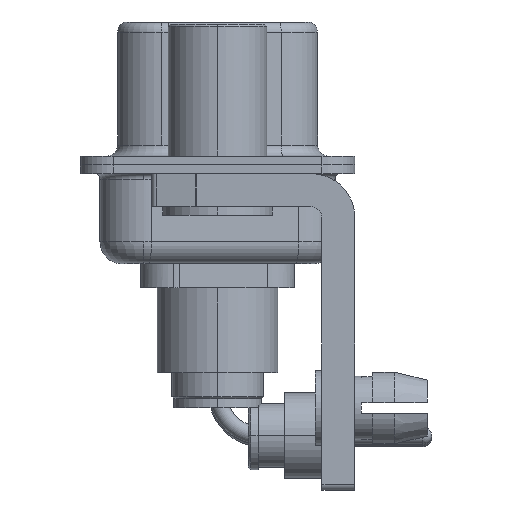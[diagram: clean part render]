
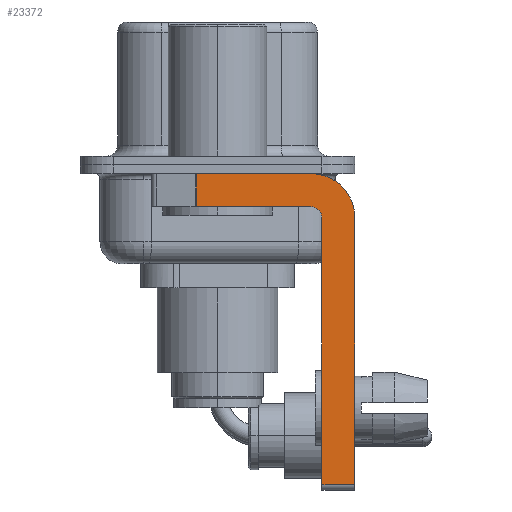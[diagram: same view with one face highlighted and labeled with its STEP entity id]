
A CAD part, left-side view. The second image highlights one B-rep face of the part: STEP entity #23372.
In plain terms, the highlighted planar face has unit normal (-1, 0, 0).
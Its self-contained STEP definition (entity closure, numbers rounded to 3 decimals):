
#220 = CARTESIAN_POINT ( 'NONE',  ( -2.9, -4.25, -1.9 ) ) ;
#683 = CARTESIAN_POINT ( 'NONE',  ( -2.9, -4.25, -2.4 ) ) ;
#1037 = CARTESIAN_POINT ( 'NONE',  ( -2.9, -4.75, -14.8 ) ) ;
#1614 = VERTEX_POINT ( 'NONE', #18601 ) ;
#1697 = DIRECTION ( 'NONE',  ( 0., 0., -1. ) ) ;
#1940 = ORIENTED_EDGE ( 'NONE', *, *, #13351, .T. ) ;
#2258 = DIRECTION ( 'NONE',  ( 0., -1., 0. ) ) ;
#2366 = VECTOR ( 'NONE', #3899, 1000. ) ;
#2411 = ORIENTED_EDGE ( 'NONE', *, *, #8951, .T. ) ;
#2453 = DIRECTION ( 'NONE',  ( 0., 0., -1. ) ) ;
#2888 = VECTOR ( 'NONE', #1697, 1000. ) ;
#3038 = CARTESIAN_POINT ( 'NONE',  ( -2.9, -4.75, -14.55 ) ) ;
#3170 = CARTESIAN_POINT ( 'NONE',  ( -2.9, -4.75, -2.4 ) ) ;
#3884 = CARTESIAN_POINT ( 'NONE',  ( -2.9, -4.25, -2.4 ) ) ;
#3899 = DIRECTION ( 'NONE',  ( 0., 1., 0. ) ) ;
#4109 = EDGE_LOOP ( 'NONE', ( #14324, #1940, #21962, #21634, #16506, #2411, #12765, #16739 ) ) ;
#4476 = LINE ( 'NONE', #1037, #23178 ) ;
#4547 = VERTEX_POINT ( 'NONE', #5367 ) ;
#4583 = CARTESIAN_POINT ( 'NONE',  ( -2.9, -6.25, -2.4 ) ) ;
#4943 = CARTESIAN_POINT ( 'NONE',  ( -2.9, -6.25, -2.4 ) ) ;
#5138 = CARTESIAN_POINT ( 'NONE',  ( -2.9, 0.978, -1.9 ) ) ;
#5247 = CARTESIAN_POINT ( 'NONE',  ( -2.9, -4.25, -2.4 ) ) ;
#5367 = CARTESIAN_POINT ( 'NONE',  ( -2.9, 0.978, -1.9 ) ) ;
#5424 = VERTEX_POINT ( 'NONE', #9056 ) ;
#6057 = VERTEX_POINT ( 'NONE', #7486 ) ;
#6517 = VECTOR ( 'NONE', #21369, 1000. ) ;
#7483 = AXIS2_PLACEMENT_3D ( 'NONE', #3884, #16546, #2453 ) ;
#7486 = CARTESIAN_POINT ( 'NONE',  ( -2.9, -4.25, -1.9 ) ) ;
#7916 = DIRECTION ( 'NONE',  ( -1., 0., 0. ) ) ;
#8078 = EDGE_CURVE ( 'NONE', #6057, #4547, #18110, .T. ) ;
#8243 = EDGE_CURVE ( 'NONE', #18488, #8383, #4476, .T. ) ;
#8383 = VERTEX_POINT ( 'NONE', #3170 ) ;
#8951 = EDGE_CURVE ( 'NONE', #18488, #5424, #23147, .T. ) ;
#9040 = DIRECTION ( 'NONE',  ( 0., 0., -1. ) ) ;
#9056 = CARTESIAN_POINT ( 'NONE',  ( -2.9, -6.25, -14.55 ) ) ;
#9406 = VERTEX_POINT ( 'NONE', #12655 ) ;
#9468 = DIRECTION ( 'NONE',  ( 0., 0., 1. ) ) ;
#10179 = AXIS2_PLACEMENT_3D ( 'NONE', #5247, #23237, #9040 ) ;
#10698 = PLANE ( 'NONE',  #10179 ) ;
#11589 = EDGE_CURVE ( 'NONE', #16038, #5424, #12169, .T. ) ;
#12169 = LINE ( 'NONE', #4943, #21726 ) ;
#12655 = CARTESIAN_POINT ( 'NONE',  ( -2.9, -4.25, -0.4 ) ) ;
#12765 = ORIENTED_EDGE ( 'NONE', *, *, #11589, .F. ) ;
#13351 = EDGE_CURVE ( 'NONE', #1614, #4547, #21689, .T. ) ;
#13500 = VECTOR ( 'NONE', #2258, 1000. ) ;
#14148 = CARTESIAN_POINT ( 'NONE',  ( -2.9, -4.25, -14.55 ) ) ;
#14324 = ORIENTED_EDGE ( 'NONE', *, *, #21709, .F. ) ;
#15143 = LINE ( 'NONE', #16702, #13500 ) ;
#15465 = DIRECTION ( 'NONE',  ( 0., 0., -1. ) ) ;
#15849 = EDGE_CURVE ( 'NONE', #9406, #16038, #17685, .T. ) ;
#16038 = VERTEX_POINT ( 'NONE', #4583 ) ;
#16506 = ORIENTED_EDGE ( 'NONE', *, *, #8243, .F. ) ;
#16546 = DIRECTION ( 'NONE',  ( 1., 0., 0. ) ) ;
#16702 = CARTESIAN_POINT ( 'NONE',  ( -2.9, 3., -0.4 ) ) ;
#16739 = ORIENTED_EDGE ( 'NONE', *, *, #15849, .F. ) ;
#17302 = CIRCLE ( 'NONE', #20344, 0.5 ) ;
#17685 = CIRCLE ( 'NONE', #7483, 2. ) ;
#18110 = LINE ( 'NONE', #220, #2366 ) ;
#18488 = VERTEX_POINT ( 'NONE', #3038 ) ;
#18601 = CARTESIAN_POINT ( 'NONE',  ( -2.9, 0.978, -0.4 ) ) ;
#19917 = FACE_OUTER_BOUND ( 'NONE', #4109, .T. ) ;
#20344 = AXIS2_PLACEMENT_3D ( 'NONE', #683, #7916, #9468 ) ;
#21369 = DIRECTION ( 'NONE',  ( 0., -1., 0. ) ) ;
#21634 = ORIENTED_EDGE ( 'NONE', *, *, #22163, .F. ) ;
#21689 = LINE ( 'NONE', #5138, #2888 ) ;
#21709 = EDGE_CURVE ( 'NONE', #1614, #9406, #15143, .T. ) ;
#21726 = VECTOR ( 'NONE', #15465, 1000. ) ;
#21962 = ORIENTED_EDGE ( 'NONE', *, *, #8078, .F. ) ;
#22163 = EDGE_CURVE ( 'NONE', #8383, #6057, #17302, .T. ) ;
#22230 = DIRECTION ( 'NONE',  ( 0., 0., 1. ) ) ;
#23147 = LINE ( 'NONE', #14148, #6517 ) ;
#23178 = VECTOR ( 'NONE', #22230, 1000. ) ;
#23237 = DIRECTION ( 'NONE',  ( 1., 0., 0. ) ) ;
#23372 = ADVANCED_FACE ( 'NONE', ( #19917 ), #10698, .F. ) ;
